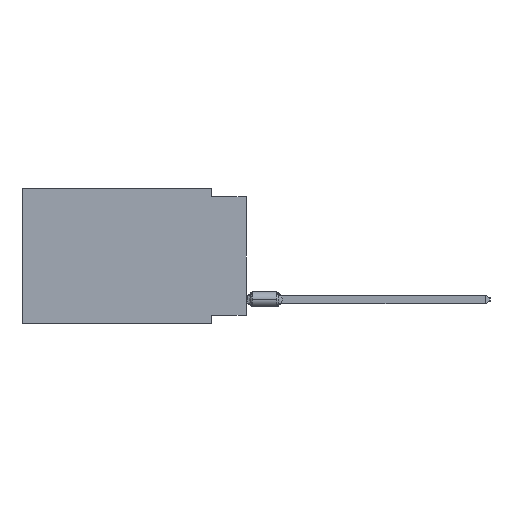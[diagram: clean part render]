
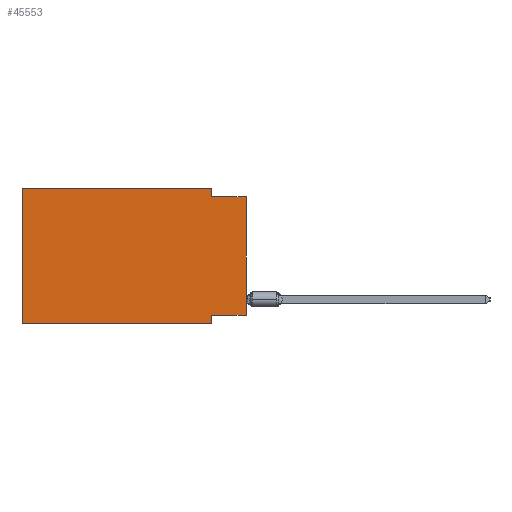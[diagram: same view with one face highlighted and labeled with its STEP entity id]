
A CAD part, left-side view. The second image highlights one B-rep face of the part: STEP entity #45553.
In plain terms, the highlighted planar face has unit normal (-1, 0, 0).
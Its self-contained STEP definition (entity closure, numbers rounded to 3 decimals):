
#438 = ORIENTED_EDGE ( 'NONE', *, *, #38797, .F. ) ;
#1239 = DIRECTION ( 'NONE',  ( 0., 0., -1. ) ) ;
#1516 = ORIENTED_EDGE ( 'NONE', *, *, #14980, .F. ) ;
#2188 = LINE ( 'NONE', #25587, #32657 ) ;
#2482 = DIRECTION ( 'NONE',  ( 0., 0., 1. ) ) ;
#3041 = EDGE_CURVE ( 'NONE', #41790, #43433, #42842, .T. ) ;
#3428 = EDGE_CURVE ( 'NONE', #10333, #22619, #9025, .T. ) ;
#3611 = CARTESIAN_POINT ( 'NONE',  ( 0., 2.54, -0.635 ) ) ;
#3644 = CARTESIAN_POINT ( 'NONE',  ( 0., 2.54, -9.906 ) ) ;
#5213 = ORIENTED_EDGE ( 'NONE', *, *, #10046, .T. ) ;
#5735 = LINE ( 'NONE', #21114, #33285 ) ;
#7311 = LINE ( 'NONE', #23433, #37626 ) ;
#8989 = VECTOR ( 'NONE', #36607, 1000. ) ;
#9025 = LINE ( 'NONE', #35472, #47633 ) ;
#10046 = EDGE_CURVE ( 'NONE', #24348, #36363, #5735, .T. ) ;
#10333 = VERTEX_POINT ( 'NONE', #44440 ) ;
#12118 = ORIENTED_EDGE ( 'NONE', *, *, #3428, .F. ) ;
#12615 = VECTOR ( 'NONE', #21183, 1000. ) ;
#13490 = VERTEX_POINT ( 'NONE', #3644 ) ;
#14980 = EDGE_CURVE ( 'NONE', #19779, #13490, #7311, .T. ) ;
#15019 = FACE_OUTER_BOUND ( 'NONE', #49182, .T. ) ;
#15258 = PLANE ( 'NONE',  #40291 ) ;
#15518 = CARTESIAN_POINT ( 'NONE',  ( 0., 16.383, 0. ) ) ;
#16039 = ORIENTED_EDGE ( 'NONE', *, *, #36221, .T. ) ;
#16281 = VECTOR ( 'NONE', #20921, 1000. ) ;
#18605 = ORIENTED_EDGE ( 'NONE', *, *, #3041, .F. ) ;
#18860 = VECTOR ( 'NONE', #26876, 1000. ) ;
#19160 = CARTESIAN_POINT ( 'NONE',  ( 0., 0., -9.271 ) ) ;
#19779 = VERTEX_POINT ( 'NONE', #38721 ) ;
#20921 = DIRECTION ( 'NONE',  ( 0., 0., 1. ) ) ;
#21114 = CARTESIAN_POINT ( 'NONE',  ( 0., 0., 0. ) ) ;
#21183 = DIRECTION ( 'NONE',  ( 0., -1., 0. ) ) ;
#22322 = CARTESIAN_POINT ( 'NONE',  ( 0., 16.383, -9.906 ) ) ;
#22619 = VERTEX_POINT ( 'NONE', #3611 ) ;
#22685 = DIRECTION ( 'NONE',  ( 0., 0., -1. ) ) ;
#23063 = DIRECTION ( 'NONE',  ( 1., 0., 0. ) ) ;
#23433 = CARTESIAN_POINT ( 'NONE',  ( 0., 2.54, -9.906 ) ) ;
#23660 = ORIENTED_EDGE ( 'NONE', *, *, #27452, .F. ) ;
#24348 = VERTEX_POINT ( 'NONE', #19160 ) ;
#25587 = CARTESIAN_POINT ( 'NONE',  ( 0., 16.383, -9.906 ) ) ;
#26618 = CARTESIAN_POINT ( 'NONE',  ( 0., 0., -0.635 ) ) ;
#26820 = CARTESIAN_POINT ( 'NONE',  ( 0., 0., -0.635 ) ) ;
#26876 = DIRECTION ( 'NONE',  ( 0., -1., 0. ) ) ;
#27452 = EDGE_CURVE ( 'NONE', #24348, #19779, #32844, .T. ) ;
#29547 = CARTESIAN_POINT ( 'NONE',  ( 0., 0., -9.271 ) ) ;
#30704 = ORIENTED_EDGE ( 'NONE', *, *, #40401, .F. ) ;
#30856 = DIRECTION ( 'NONE',  ( 0., 0., -1. ) ) ;
#32645 = DIRECTION ( 'NONE',  ( 0., -1., 0. ) ) ;
#32657 = VECTOR ( 'NONE', #32645, 1000. ) ;
#32844 = LINE ( 'NONE', #29547, #8989 ) ;
#33285 = VECTOR ( 'NONE', #2482, 1000. ) ;
#33734 = CARTESIAN_POINT ( 'NONE',  ( 0., 16.383, 0. ) ) ;
#34169 = LINE ( 'NONE', #26618, #18860 ) ;
#35281 = CARTESIAN_POINT ( 'NONE',  ( 0., 16.383, 0. ) ) ;
#35472 = CARTESIAN_POINT ( 'NONE',  ( 0., 2.54, 0. ) ) ;
#36221 = EDGE_CURVE ( 'NONE', #41790, #13490, #2188, .T. ) ;
#36363 = VERTEX_POINT ( 'NONE', #26820 ) ;
#36607 = DIRECTION ( 'NONE',  ( 0., 1., 0. ) ) ;
#37626 = VECTOR ( 'NONE', #22685, 1000. ) ;
#37854 = CARTESIAN_POINT ( 'NONE',  ( 0., 16.383, 0. ) ) ;
#38721 = CARTESIAN_POINT ( 'NONE',  ( 0., 2.54, -9.271 ) ) ;
#38797 = EDGE_CURVE ( 'NONE', #43433, #10333, #41042, .T. ) ;
#40291 = AXIS2_PLACEMENT_3D ( 'NONE', #15518, #23063, #30856 ) ;
#40401 = EDGE_CURVE ( 'NONE', #22619, #36363, #34169, .T. ) ;
#41042 = LINE ( 'NONE', #33734, #12615 ) ;
#41790 = VERTEX_POINT ( 'NONE', #22322 ) ;
#42842 = LINE ( 'NONE', #35281, #16281 ) ;
#43433 = VERTEX_POINT ( 'NONE', #37854 ) ;
#44440 = CARTESIAN_POINT ( 'NONE',  ( 0., 2.54, 0. ) ) ;
#45553 = ADVANCED_FACE ( 'NONE', ( #15019 ), #15258, .F. ) ;
#47633 = VECTOR ( 'NONE', #1239, 1000. ) ;
#49182 = EDGE_LOOP ( 'NONE', ( #5213, #30704, #12118, #438, #18605, #16039, #1516, #23660 ) ) ;
